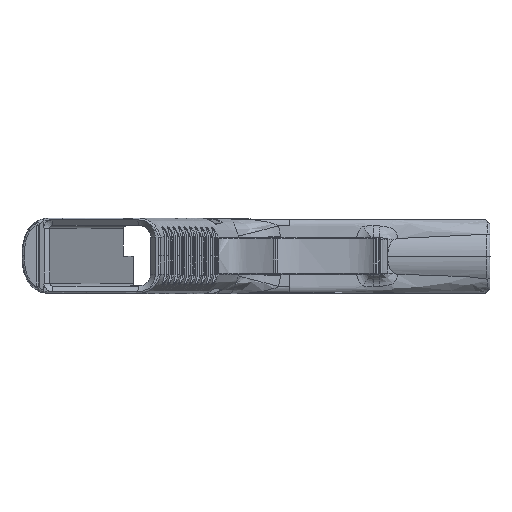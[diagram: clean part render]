
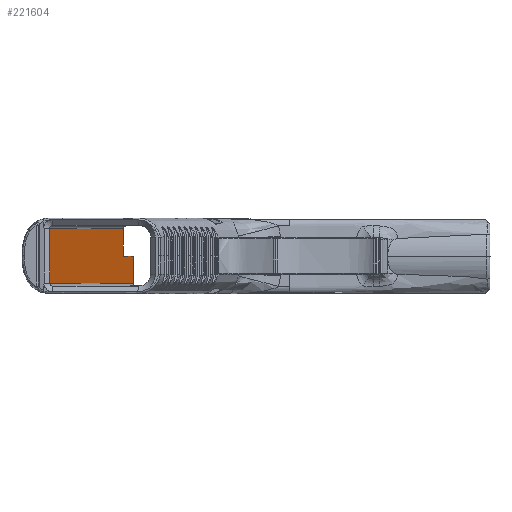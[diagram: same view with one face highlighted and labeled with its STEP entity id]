
A CAD part, top view. The second image highlights one B-rep face of the part: STEP entity #221604.
In plain terms, the highlighted planar face has unit normal (0.951, 0, 0.309).
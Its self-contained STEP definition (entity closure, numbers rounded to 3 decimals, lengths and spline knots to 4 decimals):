
#268 = VECTOR ( 'NONE', #178166, 39.3701 ) ;
#6477 = ORIENTED_EDGE ( 'NONE', *, *, #312430, .F. ) ;
#13190 = VERTEX_POINT ( 'NONE', #128618 ) ;
#22215 = LINE ( 'NONE', #317493, #26181 ) ;
#23473 = DIRECTION ( 'NONE',  ( 0., 1., 0. ) ) ;
#26181 = VECTOR ( 'NONE', #286554, 39.3701 ) ;
#30033 = VECTOR ( 'NONE', #327561, 39.3701 ) ;
#30854 = VECTOR ( 'NONE', #123861, 39.3701 ) ;
#35579 = LINE ( 'NONE', #246700, #306961 ) ;
#40378 = PLANE ( 'NONE',  #118204 ) ;
#66004 = ORIENTED_EDGE ( 'NONE', *, *, #238571, .F. ) ;
#70657 = VERTEX_POINT ( 'NONE', #85314 ) ;
#71641 = VERTEX_POINT ( 'NONE', #283446 ) ;
#74723 = FACE_OUTER_BOUND ( 'NONE', #152605, .T. ) ;
#77236 = ORIENTED_EDGE ( 'NONE', *, *, #257981, .F. ) ;
#82125 = EDGE_CURVE ( 'NONE', #71641, #187451, #312860, .T. ) ;
#85314 = CARTESIAN_POINT ( 'NONE',  ( 0.9499, 0.37, -0.4151 ) ) ;
#91525 = CARTESIAN_POINT ( 'NONE',  ( 0.9499, -0.37, -0.4151 ) ) ;
#92568 = LINE ( 'NONE', #169963, #30854 ) ;
#94514 = CARTESIAN_POINT ( 'NONE',  ( 1.9466, 0.37, -3.4826 ) ) ;
#97846 = LINE ( 'NONE', #285457, #134441 ) ;
#108758 = ORIENTED_EDGE ( 'NONE', *, *, #82125, .F. ) ;
#118204 = AXIS2_PLACEMENT_3D ( 'NONE', #118502, #225386, #144996 ) ;
#118502 = CARTESIAN_POINT ( 'NONE',  ( 2.0746, 0., -3.8765 ) ) ;
#123861 = DIRECTION ( 'NONE',  ( -0.309, 0., 0.951 ) ) ;
#128618 = CARTESIAN_POINT ( 'NONE',  ( 2.0809, -0.37, -3.896 ) ) ;
#134441 = VECTOR ( 'NONE', #23473, 39.3701 ) ;
#139116 = CARTESIAN_POINT ( 'NONE',  ( 2.0809, 0.0001, -3.896 ) ) ;
#143297 = DIRECTION ( 'NONE',  ( 0., -1., 0. ) ) ;
#144996 = DIRECTION ( 'NONE',  ( -0.309, 0., 0.951 ) ) ;
#152605 = EDGE_LOOP ( 'NONE', ( #77236, #66004, #6477, #164016, #213430, #108758 ) ) ;
#164016 = ORIENTED_EDGE ( 'NONE', *, *, #169069, .F. ) ;
#169069 = EDGE_CURVE ( 'NONE', #13190, #222507, #92568, .T. ) ;
#169963 = CARTESIAN_POINT ( 'NONE',  ( 2.0746, -0.37, -3.8765 ) ) ;
#172372 = CARTESIAN_POINT ( 'NONE',  ( 1.9466, 0., -3.4826 ) ) ;
#178166 = DIRECTION ( 'NONE',  ( 0.309, 0., -0.951 ) ) ;
#187451 = VERTEX_POINT ( 'NONE', #139116 ) ;
#212987 = EDGE_CURVE ( 'NONE', #187451, #13190, #35579, .T. ) ;
#213430 = ORIENTED_EDGE ( 'NONE', *, *, #212987, .F. ) ;
#221604 = ADVANCED_FACE ( 'NONE', ( #74723 ), #40378, .F. ) ;
#222507 = VERTEX_POINT ( 'NONE', #91525 ) ;
#223278 = LINE ( 'NONE', #172372, #30033 ) ;
#225386 = DIRECTION ( 'NONE',  ( -0.951, 0., -0.309 ) ) ;
#238571 = EDGE_CURVE ( 'NONE', #70657, #291849, #22215, .T. ) ;
#246700 = CARTESIAN_POINT ( 'NONE',  ( 2.0809, 0., -3.896 ) ) ;
#257981 = EDGE_CURVE ( 'NONE', #291849, #71641, #223278, .T. ) ;
#283446 = CARTESIAN_POINT ( 'NONE',  ( 1.9466, 0.0001, -3.4826 ) ) ;
#285457 = CARTESIAN_POINT ( 'NONE',  ( 0.9499, 0., -0.4151 ) ) ;
#286554 = DIRECTION ( 'NONE',  ( 0.309, 0., -0.951 ) ) ;
#291849 = VERTEX_POINT ( 'NONE', #94514 ) ;
#306961 = VECTOR ( 'NONE', #143297, 39.3701 ) ;
#309159 = CARTESIAN_POINT ( 'NONE',  ( 2.0746, 0.0001, -3.8765 ) ) ;
#312430 = EDGE_CURVE ( 'NONE', #222507, #70657, #97846, .T. ) ;
#312860 = LINE ( 'NONE', #309159, #268 ) ;
#317493 = CARTESIAN_POINT ( 'NONE',  ( 2.0746, 0.37, -3.8765 ) ) ;
#327561 = DIRECTION ( 'NONE',  ( 0., -1., 0. ) ) ;
